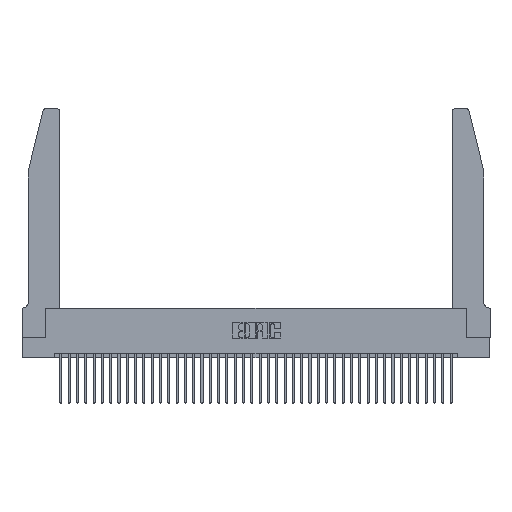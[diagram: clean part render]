
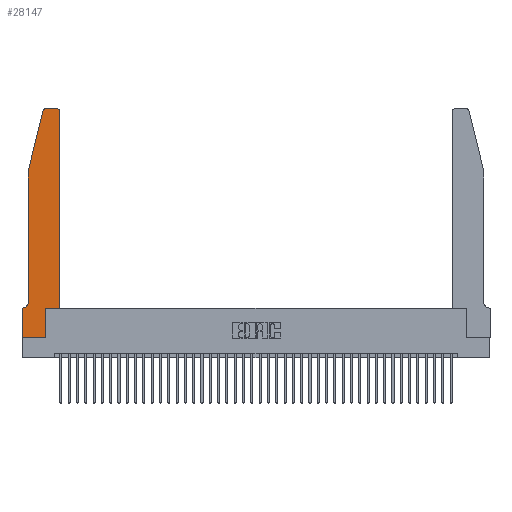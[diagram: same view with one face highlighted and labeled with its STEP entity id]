
A CAD part, top view. The second image highlights one B-rep face of the part: STEP entity #28147.
In plain terms, the highlighted planar face has unit normal (0, 0, 1).
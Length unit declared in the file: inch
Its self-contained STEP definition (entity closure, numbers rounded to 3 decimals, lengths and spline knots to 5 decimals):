
#662 = EDGE_CURVE ( 'NONE', #25375, #5251, #38698, .T. ) ;
#778 = ORIENTED_EDGE ( 'NONE', *, *, #3024, .T. ) ;
#1090 = CARTESIAN_POINT ( 'NONE',  ( 0.0755, 2., 0.37 ) ) ;
#1816 = VECTOR ( 'NONE', #29875, 39.37008 ) ;
#1980 = VECTOR ( 'NONE', #28593, 39.37008 ) ;
#2265 = EDGE_CURVE ( 'NONE', #38796, #32893, #11859, .T. ) ;
#2369 = EDGE_CURVE ( 'NONE', #8400, #41122, #26370, .T. ) ;
#2786 = CARTESIAN_POINT ( 'NONE',  ( 0.4505, 0.35, 0.37 ) ) ;
#2827 = EDGE_CURVE ( 'NONE', #3066, #23269, #38020, .T. ) ;
#3024 = EDGE_CURVE ( 'NONE', #22046, #25375, #7782, .T. ) ;
#3066 = VERTEX_POINT ( 'NONE', #12232 ) ;
#3703 = EDGE_LOOP ( 'NONE', ( #8270, #10308, #32430, #29445, #19035, #5217, #32161, #21418, #778, #26696, #31670, #18858 ) ) ;
#4232 = DIRECTION ( 'NONE',  ( 1., 0., 0. ) ) ;
#4537 = DIRECTION ( 'NONE',  ( -1., 0., 0. ) ) ;
#4930 = DIRECTION ( 'NONE',  ( 0., -1., 0. ) ) ;
#5014 = CARTESIAN_POINT ( 'NONE',  ( 0.284, 2.75, 0.37 ) ) ;
#5107 = CARTESIAN_POINT ( 'NONE',  ( 0.4205, 2.75, 0.37 ) ) ;
#5217 = ORIENTED_EDGE ( 'NONE', *, *, #11924, .T. ) ;
#5251 = VERTEX_POINT ( 'NONE', #24097 ) ;
#5469 = CARTESIAN_POINT ( 'NONE',  ( 0.2865, 0., 0.37 ) ) ;
#5501 = CARTESIAN_POINT ( 'NONE',  ( 0.2865, 0.35, 0.37 ) ) ;
#5998 = CARTESIAN_POINT ( 'NONE',  ( 0.25487, 2.72718, 0.37 ) ) ;
#7782 = LINE ( 'NONE', #5501, #18329 ) ;
#7818 = VECTOR ( 'NONE', #15207, 39.37008 ) ;
#7853 = CARTESIAN_POINT ( 'NONE',  ( 0.2605, 2.75, 0.37 ) ) ;
#8270 = ORIENTED_EDGE ( 'NONE', *, *, #2265, .T. ) ;
#8400 = VERTEX_POINT ( 'NONE', #5998 ) ;
#8615 = DIRECTION ( 'NONE',  ( 1., 0., 0. ) ) ;
#8787 = EDGE_CURVE ( 'NONE', #35052, #38796, #35573, .T. ) ;
#9677 = AXIS2_PLACEMENT_3D ( 'NONE', #29629, #39687, #4232 ) ;
#10308 = ORIENTED_EDGE ( 'NONE', *, *, #11277, .T. ) ;
#10863 = AXIS2_PLACEMENT_3D ( 'NONE', #26821, #30082, #4537 ) ;
#11277 = EDGE_CURVE ( 'NONE', #32893, #8400, #31841, .T. ) ;
#11859 = LINE ( 'NONE', #7853, #1816 ) ;
#11863 = EDGE_CURVE ( 'NONE', #23269, #22046, #20687, .T. ) ;
#11895 = AXIS2_PLACEMENT_3D ( 'NONE', #32702, #29600, #13450 ) ;
#11924 = EDGE_CURVE ( 'NONE', #30975, #3066, #17172, .T. ) ;
#11998 = CARTESIAN_POINT ( 'NONE',  ( 0., 0., 0.37 ) ) ;
#12232 = CARTESIAN_POINT ( 'NONE',  ( 0., 0.35, 0.37 ) ) ;
#13450 = DIRECTION ( 'NONE',  ( 1., 0., 0. ) ) ;
#15207 = DIRECTION ( 'NONE',  ( 0., -1., 0. ) ) ;
#16633 = VECTOR ( 'NONE', #20363, 39.37008 ) ;
#16661 = VERTEX_POINT ( 'NONE', #25727 ) ;
#17172 = LINE ( 'NONE', #29156, #18702 ) ;
#17565 = CARTESIAN_POINT ( 'NONE',  ( 0., 0., 0.37 ) ) ;
#18329 = VECTOR ( 'NONE', #21496, 39.37008 ) ;
#18490 = CARTESIAN_POINT ( 'NONE',  ( 0.0755, 2., 0.37 ) ) ;
#18702 = VECTOR ( 'NONE', #35897, 39.37008 ) ;
#18858 = ORIENTED_EDGE ( 'NONE', *, *, #8787, .T. ) ;
#19027 = CIRCLE ( 'NONE', #10863, 0.07 ) ;
#19035 = ORIENTED_EDGE ( 'NONE', *, *, #38766, .T. ) ;
#20363 = DIRECTION ( 'NONE',  ( 1., 0., 0. ) ) ;
#20687 = LINE ( 'NONE', #17565, #16633 ) ;
#20803 = CARTESIAN_POINT ( 'NONE',  ( 0., 0., 0.37 ) ) ;
#21094 = EDGE_CURVE ( 'NONE', #5251, #35052, #28391, .T. ) ;
#21418 = ORIENTED_EDGE ( 'NONE', *, *, #11863, .T. ) ;
#21496 = DIRECTION ( 'NONE',  ( 0., 1., 0. ) ) ;
#21650 = CARTESIAN_POINT ( 'NONE',  ( 0., 0.35, 0.37 ) ) ;
#22046 = VERTEX_POINT ( 'NONE', #5469 ) ;
#23269 = VERTEX_POINT ( 'NONE', #20803 ) ;
#24097 = CARTESIAN_POINT ( 'NONE',  ( 0.4505, 0.35, 0.37 ) ) ;
#25375 = VERTEX_POINT ( 'NONE', #27980 ) ;
#25727 = CARTESIAN_POINT ( 'NONE',  ( 0.0755, 0.42, 0.37 ) ) ;
#26370 = LINE ( 'NONE', #18490, #40594 ) ;
#26696 = ORIENTED_EDGE ( 'NONE', *, *, #662, .T. ) ;
#26804 = DIRECTION ( 'NONE',  ( 0., 1., 0. ) ) ;
#26821 = CARTESIAN_POINT ( 'NONE',  ( 0.0055, 0.42, 0.37 ) ) ;
#27970 = PLANE ( 'NONE',  #28986 ) ;
#27980 = CARTESIAN_POINT ( 'NONE',  ( 0.2865, 0.35, 0.37 ) ) ;
#28147 = ADVANCED_FACE ( 'NONE', ( #32038 ), #27970, .T. ) ;
#28391 = LINE ( 'NONE', #36406, #38532 ) ;
#28593 = DIRECTION ( 'NONE',  ( 1., 0., 0. ) ) ;
#28986 = AXIS2_PLACEMENT_3D ( 'NONE', #21650, #37566, #8615 ) ;
#29156 = CARTESIAN_POINT ( 'NONE',  ( 0.0755, 0.35, 0.37 ) ) ;
#29445 = ORIENTED_EDGE ( 'NONE', *, *, #39568, .T. ) ;
#29600 = DIRECTION ( 'NONE',  ( 0., 0., 1. ) ) ;
#29629 = CARTESIAN_POINT ( 'NONE',  ( 0.4205, 2.72, 0.37 ) ) ;
#29875 = DIRECTION ( 'NONE',  ( -1., 0., 0. ) ) ;
#30082 = DIRECTION ( 'NONE',  ( 0., 0., -1. ) ) ;
#30411 = CARTESIAN_POINT ( 'NONE',  ( 0.4505, 2.72, 0.37 ) ) ;
#30975 = VERTEX_POINT ( 'NONE', #37218 ) ;
#31670 = ORIENTED_EDGE ( 'NONE', *, *, #21094, .T. ) ;
#31841 = CIRCLE ( 'NONE', #11895, 0.03 ) ;
#32038 = FACE_OUTER_BOUND ( 'NONE', #3703, .T. ) ;
#32161 = ORIENTED_EDGE ( 'NONE', *, *, #2827, .T. ) ;
#32430 = ORIENTED_EDGE ( 'NONE', *, *, #2369, .T. ) ;
#32702 = CARTESIAN_POINT ( 'NONE',  ( 0.284, 2.72, 0.37 ) ) ;
#32893 = VERTEX_POINT ( 'NONE', #5014 ) ;
#35052 = VERTEX_POINT ( 'NONE', #30411 ) ;
#35088 = LINE ( 'NONE', #40662, #41164 ) ;
#35573 = CIRCLE ( 'NONE', #9677, 0.03 ) ;
#35897 = DIRECTION ( 'NONE',  ( -1., 0., 0. ) ) ;
#36406 = CARTESIAN_POINT ( 'NONE',  ( 0.4505, 0.35, 0.37 ) ) ;
#37218 = CARTESIAN_POINT ( 'NONE',  ( 0.0055, 0.35, 0.37 ) ) ;
#37566 = DIRECTION ( 'NONE',  ( 0., 0., 1. ) ) ;
#38020 = LINE ( 'NONE', #11998, #7818 ) ;
#38532 = VECTOR ( 'NONE', #26804, 39.37008 ) ;
#38698 = LINE ( 'NONE', #2786, #1980 ) ;
#38766 = EDGE_CURVE ( 'NONE', #16661, #30975, #19027, .T. ) ;
#38796 = VERTEX_POINT ( 'NONE', #5107 ) ;
#39568 = EDGE_CURVE ( 'NONE', #41122, #16661, #35088, .T. ) ;
#39687 = DIRECTION ( 'NONE',  ( 0., 0., 1. ) ) ;
#40594 = VECTOR ( 'NONE', #41057, 39.37008 ) ;
#40662 = CARTESIAN_POINT ( 'NONE',  ( 0.0755, 2., 0.37 ) ) ;
#41057 = DIRECTION ( 'NONE',  ( -0.239, -0.971, 0. ) ) ;
#41122 = VERTEX_POINT ( 'NONE', #1090 ) ;
#41164 = VECTOR ( 'NONE', #4930, 39.37008 ) ;
